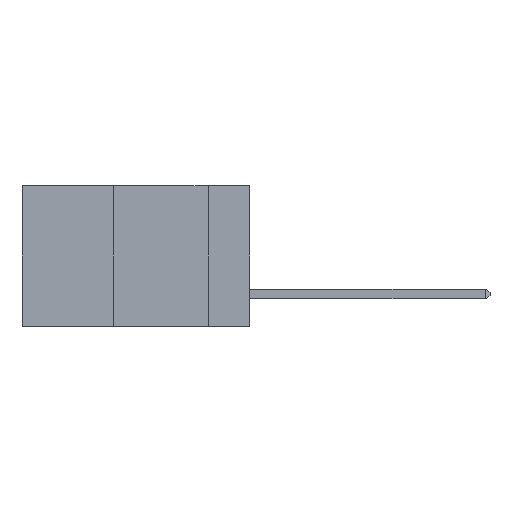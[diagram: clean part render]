
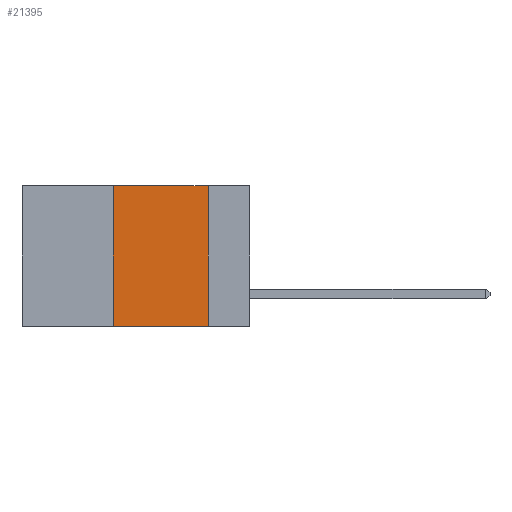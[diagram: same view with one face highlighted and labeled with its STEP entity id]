
A CAD part, left-side view. The second image highlights one B-rep face of the part: STEP entity #21395.
In plain terms, the highlighted planar face has unit normal (-1, 0, 0).
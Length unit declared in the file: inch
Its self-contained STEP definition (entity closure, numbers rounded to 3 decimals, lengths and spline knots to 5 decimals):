
#727 = EDGE_CURVE ( 'NONE', #13247, #8900, #6422, .T. ) ;
#1157 = CARTESIAN_POINT ( 'NONE',  ( 0., 0.36, -0.37 ) ) ;
#1238 = DIRECTION ( 'NONE',  ( 0., 0., -1. ) ) ;
#1605 = EDGE_CURVE ( 'NONE', #13247, #16905, #10589, .T. ) ;
#1782 = VECTOR ( 'NONE', #17089, 39.37008 ) ;
#2283 = PLANE ( 'NONE',  #6858 ) ;
#6134 = EDGE_CURVE ( 'NONE', #8900, #10186, #12139, .T. ) ;
#6320 = ORIENTED_EDGE ( 'NONE', *, *, #1605, .T. ) ;
#6388 = EDGE_LOOP ( 'NONE', ( #14772, #24851, #10845, #6320 ) ) ;
#6422 = LINE ( 'NONE', #24930, #21729 ) ;
#6858 = AXIS2_PLACEMENT_3D ( 'NONE', #11994, #19687, #8226 ) ;
#8226 = DIRECTION ( 'NONE',  ( 0., 0., -1. ) ) ;
#8900 = VERTEX_POINT ( 'NONE', #14736 ) ;
#9353 = CARTESIAN_POINT ( 'NONE',  ( 0., 0.6, 0. ) ) ;
#9655 = FACE_OUTER_BOUND ( 'NONE', #6388, .T. ) ;
#10186 = VERTEX_POINT ( 'NONE', #22676 ) ;
#10589 = LINE ( 'NONE', #11286, #15701 ) ;
#10845 = ORIENTED_EDGE ( 'NONE', *, *, #727, .F. ) ;
#11286 = CARTESIAN_POINT ( 'NONE',  ( 0., 0.6, -0.37 ) ) ;
#11775 = DIRECTION ( 'NONE',  ( 0., -1., 0. ) ) ;
#11994 = CARTESIAN_POINT ( 'NONE',  ( 0., 0.6, 0. ) ) ;
#12139 = LINE ( 'NONE', #9353, #1782 ) ;
#13247 = VERTEX_POINT ( 'NONE', #1157 ) ;
#13282 = EDGE_CURVE ( 'NONE', #10186, #16905, #16274, .T. ) ;
#14736 = CARTESIAN_POINT ( 'NONE',  ( 0., 0.36, 0. ) ) ;
#14772 = ORIENTED_EDGE ( 'NONE', *, *, #13282, .F. ) ;
#14842 = CARTESIAN_POINT ( 'NONE',  ( 0., 0.11, 0. ) ) ;
#15701 = VECTOR ( 'NONE', #11775, 39.37008 ) ;
#15774 = CARTESIAN_POINT ( 'NONE',  ( 0., 0.11, -0.37 ) ) ;
#16274 = LINE ( 'NONE', #14842, #20750 ) ;
#16905 = VERTEX_POINT ( 'NONE', #15774 ) ;
#17089 = DIRECTION ( 'NONE',  ( 0., -1., 0. ) ) ;
#19687 = DIRECTION ( 'NONE',  ( 1., 0., 0. ) ) ;
#20750 = VECTOR ( 'NONE', #1238, 39.37008 ) ;
#21395 = ADVANCED_FACE ( 'NONE', ( #9655 ), #2283, .F. ) ;
#21729 = VECTOR ( 'NONE', #24145, 39.37008 ) ;
#22676 = CARTESIAN_POINT ( 'NONE',  ( 0., 0.11, 0. ) ) ;
#24145 = DIRECTION ( 'NONE',  ( 0., 0., 1. ) ) ;
#24851 = ORIENTED_EDGE ( 'NONE', *, *, #6134, .F. ) ;
#24930 = CARTESIAN_POINT ( 'NONE',  ( 0., 0.36, 0. ) ) ;
